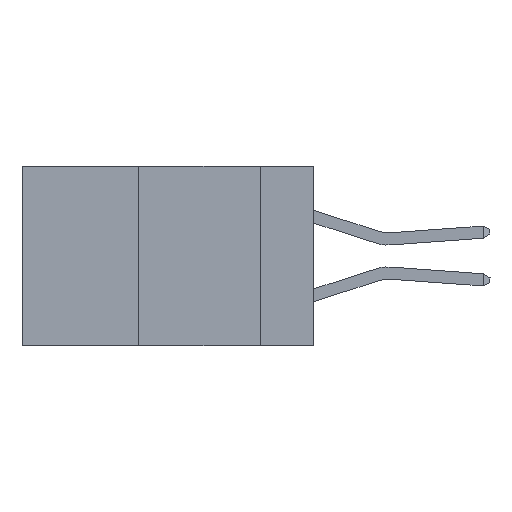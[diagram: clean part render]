
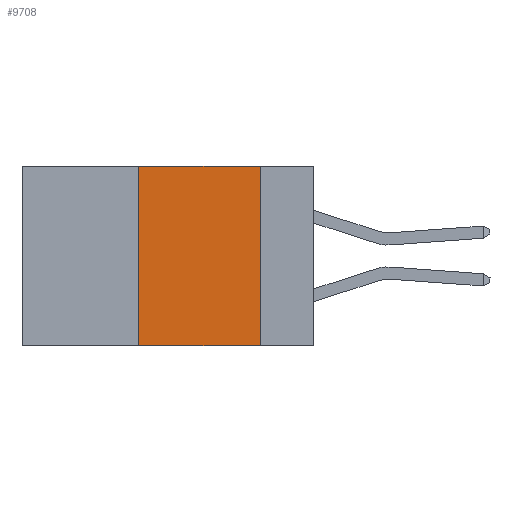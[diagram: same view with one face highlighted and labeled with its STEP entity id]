
A CAD part, left-side view. The second image highlights one B-rep face of the part: STEP entity #9708.
In plain terms, the highlighted planar face has unit normal (-1, 0, 0).
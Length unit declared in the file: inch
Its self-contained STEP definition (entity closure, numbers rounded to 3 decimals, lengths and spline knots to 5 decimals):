
#1262 = CARTESIAN_POINT ( 'NONE',  ( 0., 0.6, -0.37 ) ) ;
#1696 = EDGE_CURVE ( 'NONE', #14189, #6014, #8279, .T. ) ;
#2407 = VECTOR ( 'NONE', #9252, 39.37008 ) ;
#2697 = LINE ( 'NONE', #1262, #9819 ) ;
#2870 = LINE ( 'NONE', #13451, #2407 ) ;
#4530 = VECTOR ( 'NONE', #15399, 39.37008 ) ;
#4531 = PLANE ( 'NONE',  #8283 ) ;
#5489 = CARTESIAN_POINT ( 'NONE',  ( 0., 0.11, 0. ) ) ;
#5623 = FACE_OUTER_BOUND ( 'NONE', #7397, .T. ) ;
#5683 = CARTESIAN_POINT ( 'NONE',  ( 0., 0.36, 0. ) ) ;
#5965 = DIRECTION ( 'NONE',  ( 1., 0., 0. ) ) ;
#6014 = VERTEX_POINT ( 'NONE', #11312 ) ;
#6508 = EDGE_CURVE ( 'NONE', #6935, #10417, #17812, .T. ) ;
#6813 = VECTOR ( 'NONE', #9572, 39.37008 ) ;
#6935 = VERTEX_POINT ( 'NONE', #5489 ) ;
#7397 = EDGE_LOOP ( 'NONE', ( #11630, #12144, #13292, #13989 ) ) ;
#8145 = CARTESIAN_POINT ( 'NONE',  ( 0., 0.11, 0. ) ) ;
#8279 = LINE ( 'NONE', #5683, #4530 ) ;
#8283 = AXIS2_PLACEMENT_3D ( 'NONE', #12955, #5965, #15666 ) ;
#9252 = DIRECTION ( 'NONE',  ( 0., -1., 0. ) ) ;
#9572 = DIRECTION ( 'NONE',  ( 0., 0., -1. ) ) ;
#9676 = EDGE_CURVE ( 'NONE', #14189, #10417, #2697, .T. ) ;
#9681 = CARTESIAN_POINT ( 'NONE',  ( 0., 0.11, -0.37 ) ) ;
#9708 = ADVANCED_FACE ( 'NONE', ( #5623 ), #4531, .F. ) ;
#9819 = VECTOR ( 'NONE', #14039, 39.37008 ) ;
#10417 = VERTEX_POINT ( 'NONE', #9681 ) ;
#11312 = CARTESIAN_POINT ( 'NONE',  ( 0., 0.36, 0. ) ) ;
#11630 = ORIENTED_EDGE ( 'NONE', *, *, #6508, .F. ) ;
#12144 = ORIENTED_EDGE ( 'NONE', *, *, #13852, .F. ) ;
#12955 = CARTESIAN_POINT ( 'NONE',  ( 0., 0.6, 0. ) ) ;
#13292 = ORIENTED_EDGE ( 'NONE', *, *, #1696, .F. ) ;
#13451 = CARTESIAN_POINT ( 'NONE',  ( 0., 0.6, 0. ) ) ;
#13852 = EDGE_CURVE ( 'NONE', #6014, #6935, #2870, .T. ) ;
#13989 = ORIENTED_EDGE ( 'NONE', *, *, #9676, .T. ) ;
#14039 = DIRECTION ( 'NONE',  ( 0., -1., 0. ) ) ;
#14189 = VERTEX_POINT ( 'NONE', #15554 ) ;
#15399 = DIRECTION ( 'NONE',  ( 0., 0., 1. ) ) ;
#15554 = CARTESIAN_POINT ( 'NONE',  ( 0., 0.36, -0.37 ) ) ;
#15666 = DIRECTION ( 'NONE',  ( 0., 0., -1. ) ) ;
#17812 = LINE ( 'NONE', #8145, #6813 ) ;
